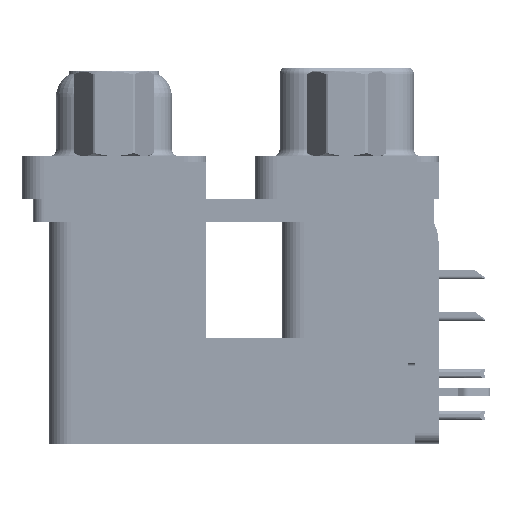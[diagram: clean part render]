
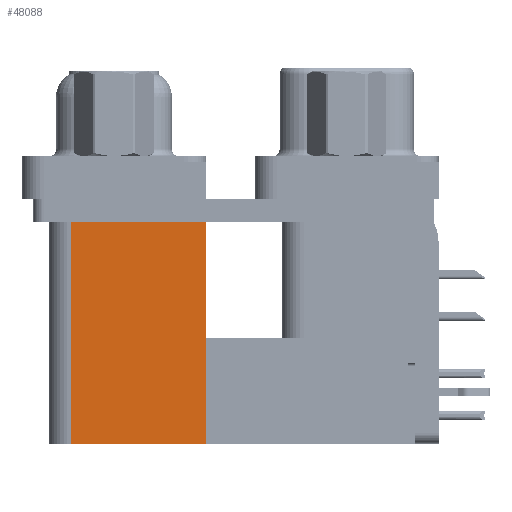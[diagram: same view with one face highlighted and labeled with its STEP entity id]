
A CAD part, left-side view. The second image highlights one B-rep face of the part: STEP entity #48088.
In plain terms, the highlighted planar face has unit normal (-1, 0, 0).
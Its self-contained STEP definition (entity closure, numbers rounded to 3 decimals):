
#3324 = VECTOR ( 'NONE', #6370, 1000. ) ;
#4500 = ORIENTED_EDGE ( 'NONE', *, *, #44588, .F. ) ;
#6370 = DIRECTION ( 'NONE',  ( 0., 1., 0. ) ) ;
#8909 = CARTESIAN_POINT ( 'NONE',  ( 3.79, 9.6, -19.2 ) ) ;
#9068 = CARTESIAN_POINT ( 'NONE',  ( 3.79, 9.6, -2.5 ) ) ;
#10122 = CARTESIAN_POINT ( 'NONE',  ( 3.79, 18.8, -19.2 ) ) ;
#12827 = LINE ( 'NONE', #64813, #41243 ) ;
#13227 = ORIENTED_EDGE ( 'NONE', *, *, #64352, .F. ) ;
#13982 = EDGE_CURVE ( 'NONE', #56739, #56087, #12827, .T. ) ;
#17615 = FACE_OUTER_BOUND ( 'NONE', #63654, .T. ) ;
#17881 = VERTEX_POINT ( 'NONE', #10122 ) ;
#21149 = CARTESIAN_POINT ( 'NONE',  ( 3.79, 9.6, -19.2 ) ) ;
#23010 = CARTESIAN_POINT ( 'NONE',  ( 3.79, 9.6, -2.5 ) ) ;
#35939 = VECTOR ( 'NONE', #46121, 1000. ) ;
#39670 = VECTOR ( 'NONE', #43898, 1000. ) ;
#40641 = LINE ( 'NONE', #23010, #3324 ) ;
#41243 = VECTOR ( 'NONE', #46722, 1000. ) ;
#42791 = DIRECTION ( 'NONE',  ( 1., 0., 0. ) ) ;
#43898 = DIRECTION ( 'NONE',  ( 0., 0., 1. ) ) ;
#44588 = EDGE_CURVE ( 'NONE', #17881, #60121, #61628, .T. ) ;
#44766 = AXIS2_PLACEMENT_3D ( 'NONE', #8909, #42791, #70303 ) ;
#46121 = DIRECTION ( 'NONE',  ( 0., 1., 0. ) ) ;
#46722 = DIRECTION ( 'NONE',  ( 0., 0., 1. ) ) ;
#48088 = ADVANCED_FACE ( 'NONE', ( #17615 ), #71056, .F. ) ;
#51782 = LINE ( 'NONE', #58190, #35939 ) ;
#55200 = ORIENTED_EDGE ( 'NONE', *, *, #13982, .T. ) ;
#56087 = VERTEX_POINT ( 'NONE', #9068 ) ;
#56739 = VERTEX_POINT ( 'NONE', #21149 ) ;
#57727 = CARTESIAN_POINT ( 'NONE',  ( 3.79, 18.8, -19.2 ) ) ;
#58190 = CARTESIAN_POINT ( 'NONE',  ( 3.79, 9.6, -19.2 ) ) ;
#58723 = ORIENTED_EDGE ( 'NONE', *, *, #61156, .T. ) ;
#60121 = VERTEX_POINT ( 'NONE', #65099 ) ;
#61156 = EDGE_CURVE ( 'NONE', #56087, #60121, #40641, .T. ) ;
#61628 = LINE ( 'NONE', #57727, #39670 ) ;
#63654 = EDGE_LOOP ( 'NONE', ( #58723, #4500, #13227, #55200 ) ) ;
#64352 = EDGE_CURVE ( 'NONE', #56739, #17881, #51782, .T. ) ;
#64813 = CARTESIAN_POINT ( 'NONE',  ( 3.79, 9.6, -19.2 ) ) ;
#65099 = CARTESIAN_POINT ( 'NONE',  ( 3.79, 18.8, -2.5 ) ) ;
#70303 = DIRECTION ( 'NONE',  ( 0., 1., 0. ) ) ;
#71056 = PLANE ( 'NONE',  #44766 ) ;
